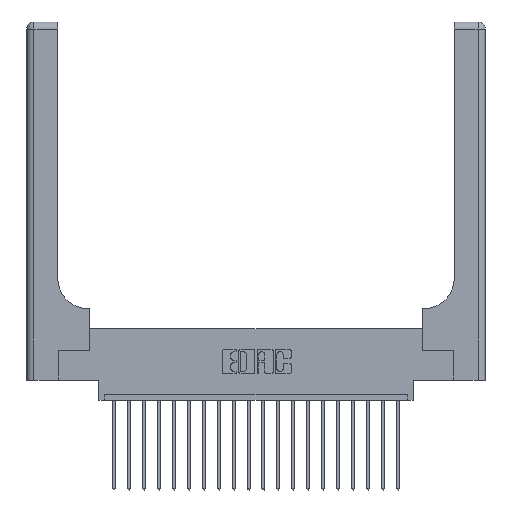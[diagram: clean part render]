
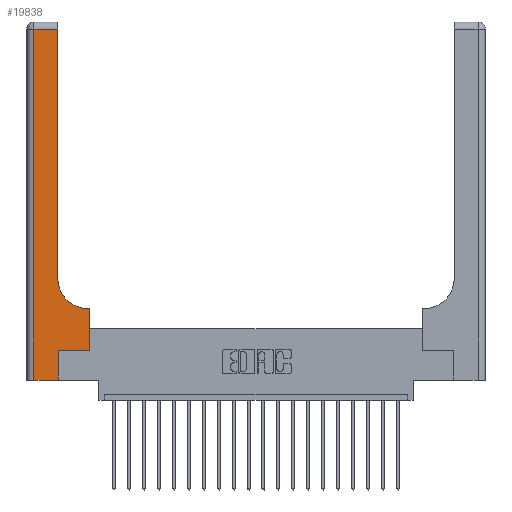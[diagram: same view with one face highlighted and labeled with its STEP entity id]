
A CAD part, top view. The second image highlights one B-rep face of the part: STEP entity #19838.
In plain terms, the highlighted planar face has unit normal (0, 0, 1).
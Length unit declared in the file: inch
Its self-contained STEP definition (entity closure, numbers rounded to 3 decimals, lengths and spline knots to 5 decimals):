
#556 = EDGE_CURVE ( 'NONE', #1800, #14997, #4268, .T. ) ;
#834 = CARTESIAN_POINT ( 'NONE',  ( 0.26, 0.85, 0.37 ) ) ;
#953 = CARTESIAN_POINT ( 'NONE',  ( 0.26, 0.6, 0.37 ) ) ;
#1247 = ORIENTED_EDGE ( 'NONE', *, *, #556, .T. ) ;
#1425 = CARTESIAN_POINT ( 'NONE',  ( 0.06, 3., 0.37 ) ) ;
#1645 = LINE ( 'NONE', #953, #16908 ) ;
#1666 = CARTESIAN_POINT ( 'NONE',  ( 0.51, 0.6, 0.37 ) ) ;
#1800 = VERTEX_POINT ( 'NONE', #834 ) ;
#2076 = DIRECTION ( 'NONE',  ( 0., 0., -1. ) ) ;
#2154 = ORIENTED_EDGE ( 'NONE', *, *, #19776, .T. ) ;
#2218 = CARTESIAN_POINT ( 'NONE',  ( 0.265, 0.25, 0.37 ) ) ;
#2345 = CARTESIAN_POINT ( 'NONE',  ( 0., 3., 0.37 ) ) ;
#2351 = DIRECTION ( 'NONE',  ( 1., 0., 0. ) ) ;
#2602 = ORIENTED_EDGE ( 'NONE', *, *, #15542, .T. ) ;
#2762 = CARTESIAN_POINT ( 'NONE',  ( 0.26, 2.94, 0.37 ) ) ;
#2791 = EDGE_CURVE ( 'NONE', #3606, #20172, #5891, .T. ) ;
#3449 = LINE ( 'NONE', #19223, #7406 ) ;
#3606 = VERTEX_POINT ( 'NONE', #8969 ) ;
#3911 = VERTEX_POINT ( 'NONE', #19166 ) ;
#3963 = ORIENTED_EDGE ( 'NONE', *, *, #5936, .T. ) ;
#4001 = DIRECTION ( 'NONE',  ( 0., 0., -1. ) ) ;
#4008 = DIRECTION ( 'NONE',  ( 1., 0., 0. ) ) ;
#4044 = CARTESIAN_POINT ( 'NONE',  ( 0.265, 0., 0.37 ) ) ;
#4133 = CARTESIAN_POINT ( 'NONE',  ( 0., 0., 0.37 ) ) ;
#4268 = LINE ( 'NONE', #6981, #9520 ) ;
#4356 = CARTESIAN_POINT ( 'NONE',  ( 0.528, 0.25, 0.37 ) ) ;
#4463 = LINE ( 'NONE', #12693, #12457 ) ;
#4591 = ORIENTED_EDGE ( 'NONE', *, *, #19033, .T. ) ;
#4647 = CARTESIAN_POINT ( 'NONE',  ( 0.06, 0., 0.37 ) ) ;
#5388 = CARTESIAN_POINT ( 'NONE',  ( 0.528, 0.6, 0.37 ) ) ;
#5891 = LINE ( 'NONE', #1425, #19182 ) ;
#5936 = EDGE_CURVE ( 'NONE', #3911, #16642, #16984, .T. ) ;
#6002 = LINE ( 'NONE', #4133, #12037 ) ;
#6357 = VECTOR ( 'NONE', #11607, 39.37008 ) ;
#6621 = LINE ( 'NONE', #16099, #6357 ) ;
#6981 = CARTESIAN_POINT ( 'NONE',  ( 0.26, 3., 0.37 ) ) ;
#7406 = VECTOR ( 'NONE', #9790, 39.37008 ) ;
#7599 = EDGE_CURVE ( 'NONE', #14997, #3606, #6621, .T. ) ;
#8969 = CARTESIAN_POINT ( 'NONE',  ( 0.06, 2.94, 0.37 ) ) ;
#9076 = EDGE_LOOP ( 'NONE', ( #1247, #13841, #13584, #18288, #2602, #3963, #4591, #14731, #2154 ) ) ;
#9520 = VECTOR ( 'NONE', #11810, 39.37008 ) ;
#9790 = DIRECTION ( 'NONE',  ( 0., 1., 0. ) ) ;
#10296 = DIRECTION ( 'NONE',  ( -1., 0., 0. ) ) ;
#10589 = AXIS2_PLACEMENT_3D ( 'NONE', #2345, #4001, #10296 ) ;
#10597 = VERTEX_POINT ( 'NONE', #1666 ) ;
#11607 = DIRECTION ( 'NONE',  ( -1., 0., 0. ) ) ;
#11810 = DIRECTION ( 'NONE',  ( 0., 1., 0. ) ) ;
#11832 = PLANE ( 'NONE',  #10589 ) ;
#11926 = DIRECTION ( 'NONE',  ( -1., 0., 0. ) ) ;
#12037 = VECTOR ( 'NONE', #2351, 39.37008 ) ;
#12301 = EDGE_CURVE ( 'NONE', #20172, #18775, #6002, .T. ) ;
#12457 = VECTOR ( 'NONE', #20458, 39.37008 ) ;
#12693 = CARTESIAN_POINT ( 'NONE',  ( 0.528, 0.25, 0.37 ) ) ;
#12721 = AXIS2_PLACEMENT_3D ( 'NONE', #16279, #2076, #13262 ) ;
#13262 = DIRECTION ( 'NONE',  ( 1., 0., 0. ) ) ;
#13584 = ORIENTED_EDGE ( 'NONE', *, *, #2791, .T. ) ;
#13841 = ORIENTED_EDGE ( 'NONE', *, *, #7599, .T. ) ;
#14083 = DIRECTION ( 'NONE',  ( 0., -1., 0. ) ) ;
#14731 = ORIENTED_EDGE ( 'NONE', *, *, #16549, .T. ) ;
#14997 = VERTEX_POINT ( 'NONE', #2762 ) ;
#15542 = EDGE_CURVE ( 'NONE', #18775, #3911, #3449, .T. ) ;
#16099 = CARTESIAN_POINT ( 'NONE',  ( 0., 2.94, 0.37 ) ) ;
#16279 = CARTESIAN_POINT ( 'NONE',  ( 0.51, 0.85, 0.37 ) ) ;
#16549 = EDGE_CURVE ( 'NONE', #19865, #10597, #1645, .T. ) ;
#16642 = VERTEX_POINT ( 'NONE', #4356 ) ;
#16908 = VECTOR ( 'NONE', #11926, 39.37008 ) ;
#16949 = FACE_OUTER_BOUND ( 'NONE', #9076, .T. ) ;
#16984 = LINE ( 'NONE', #2218, #17759 ) ;
#17759 = VECTOR ( 'NONE', #4008, 39.37008 ) ;
#18288 = ORIENTED_EDGE ( 'NONE', *, *, #12301, .T. ) ;
#18488 = CIRCLE ( 'NONE', #12721, 0.25 ) ;
#18775 = VERTEX_POINT ( 'NONE', #4044 ) ;
#19033 = EDGE_CURVE ( 'NONE', #16642, #19865, #4463, .T. ) ;
#19166 = CARTESIAN_POINT ( 'NONE',  ( 0.265, 0.25, 0.37 ) ) ;
#19182 = VECTOR ( 'NONE', #14083, 39.37008 ) ;
#19223 = CARTESIAN_POINT ( 'NONE',  ( 0.265, 0., 0.37 ) ) ;
#19776 = EDGE_CURVE ( 'NONE', #10597, #1800, #18488, .T. ) ;
#19838 = ADVANCED_FACE ( 'NONE', ( #16949 ), #11832, .F. ) ;
#19865 = VERTEX_POINT ( 'NONE', #5388 ) ;
#20172 = VERTEX_POINT ( 'NONE', #4647 ) ;
#20458 = DIRECTION ( 'NONE',  ( 0., 1., 0. ) ) ;
